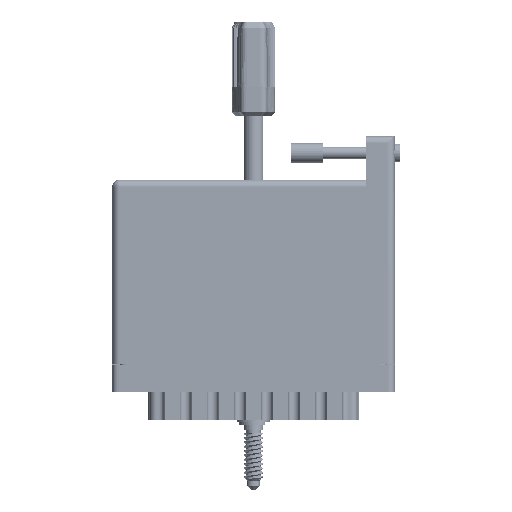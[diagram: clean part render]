
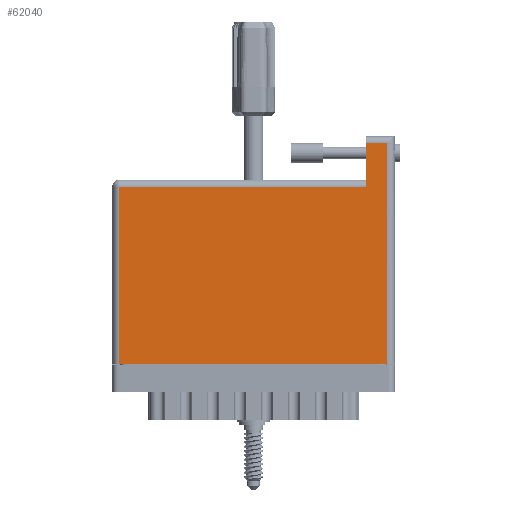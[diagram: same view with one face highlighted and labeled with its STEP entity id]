
A CAD part, front view. The second image highlights one B-rep face of the part: STEP entity #62040.
In plain terms, the highlighted face is planar.
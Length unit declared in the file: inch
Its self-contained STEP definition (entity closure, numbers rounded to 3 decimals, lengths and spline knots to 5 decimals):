
#1843 = LINE ( 'NONE', #53933, #72961 ) ;
#3958 = VERTEX_POINT ( 'NONE', #17816 ) ;
#4711 = VECTOR ( 'NONE', #77707, 39.37008 ) ;
#5452 = LINE ( 'NONE', #44135, #77604 ) ;
#7890 = CARTESIAN_POINT ( 'NONE',  ( 0., 1.775, 0. ) ) ;
#7908 = VECTOR ( 'NONE', #14143, 39.37008 ) ;
#7951 = LINE ( 'NONE', #14470, #43475 ) ;
#9631 = EDGE_CURVE ( 'NONE', #58640, #10174, #5452, .T. ) ;
#10076 = LINE ( 'NONE', #42777, #7908 ) ;
#10174 = VERTEX_POINT ( 'NONE', #40898 ) ;
#12163 = CARTESIAN_POINT ( 'NONE',  ( 2.648, 0., 0. ) ) ;
#14143 = DIRECTION ( 'NONE',  ( -1., 0., 0. ) ) ;
#14470 = CARTESIAN_POINT ( 'NONE',  ( 2.438, 2.195, 0. ) ) ;
#17816 = CARTESIAN_POINT ( 'NONE',  ( 2.438, 2.125, 0. ) ) ;
#17853 = AXIS2_PLACEMENT_3D ( 'NONE', #7890, #41314, #27472 ) ;
#20878 = LINE ( 'NONE', #71694, #4711 ) ;
#25406 = VERTEX_POINT ( 'NONE', #12163 ) ;
#27472 = DIRECTION ( 'NONE',  ( -1., 0., 0. ) ) ;
#27794 = ORIENTED_EDGE ( 'NONE', *, *, #43831, .T. ) ;
#31403 = EDGE_CURVE ( 'NONE', #37777, #58640, #10076, .T. ) ;
#35736 = CARTESIAN_POINT ( 'NONE',  ( 2.648, 2.125, 0. ) ) ;
#36382 = EDGE_CURVE ( 'NONE', #63405, #3958, #20878, .T. ) ;
#37777 = VERTEX_POINT ( 'NONE', #45306 ) ;
#40898 = CARTESIAN_POINT ( 'NONE',  ( 0.07, 0., 0. ) ) ;
#41314 = DIRECTION ( 'NONE',  ( 0., 0., -1. ) ) ;
#42777 = CARTESIAN_POINT ( 'NONE',  ( 0., 1.705, 0. ) ) ;
#43117 = FACE_OUTER_BOUND ( 'NONE', #64980, .T. ) ;
#43475 = VECTOR ( 'NONE', #55741, 39.37008 ) ;
#43831 = EDGE_CURVE ( 'NONE', #3958, #37777, #7951, .T. ) ;
#44135 = CARTESIAN_POINT ( 'NONE',  ( 0.07, 0., 0. ) ) ;
#45306 = CARTESIAN_POINT ( 'NONE',  ( 2.438, 1.705, 0. ) ) ;
#49825 = ORIENTED_EDGE ( 'NONE', *, *, #9631, .T. ) ;
#51878 = DIRECTION ( 'NONE',  ( 0., 1., 0. ) ) ;
#53933 = CARTESIAN_POINT ( 'NONE',  ( 0., 0., 0. ) ) ;
#55741 = DIRECTION ( 'NONE',  ( 0., -1., 0. ) ) ;
#57926 = DIRECTION ( 'NONE',  ( 0., -1., 0. ) ) ;
#58640 = VERTEX_POINT ( 'NONE', #62967 ) ;
#62040 = ADVANCED_FACE ( 'NONE', ( #43117 ), #69607, .F. ) ;
#62967 = CARTESIAN_POINT ( 'NONE',  ( 0.07, 1.705, 0. ) ) ;
#63405 = VERTEX_POINT ( 'NONE', #35736 ) ;
#63623 = ORIENTED_EDGE ( 'NONE', *, *, #73293, .T. ) ;
#64980 = EDGE_LOOP ( 'NONE', ( #83789, #49825, #63623, #77689, #68347, #27794 ) ) ;
#68347 = ORIENTED_EDGE ( 'NONE', *, *, #36382, .T. ) ;
#69607 = PLANE ( 'NONE',  #17853 ) ;
#71694 = CARTESIAN_POINT ( 'NONE',  ( 0., 2.125, 0. ) ) ;
#71730 = VECTOR ( 'NONE', #51878, 39.37008 ) ;
#72961 = VECTOR ( 'NONE', #81941, 39.37008 ) ;
#73293 = EDGE_CURVE ( 'NONE', #10174, #25406, #1843, .T. ) ;
#76004 = LINE ( 'NONE', #79254, #71730 ) ;
#77604 = VECTOR ( 'NONE', #57926, 39.37008 ) ;
#77689 = ORIENTED_EDGE ( 'NONE', *, *, #79903, .T. ) ;
#77707 = DIRECTION ( 'NONE',  ( -1., 0., 0. ) ) ;
#79254 = CARTESIAN_POINT ( 'NONE',  ( 2.648, 2.195, 0. ) ) ;
#79903 = EDGE_CURVE ( 'NONE', #25406, #63405, #76004, .T. ) ;
#81941 = DIRECTION ( 'NONE',  ( 1., 0., 0. ) ) ;
#83789 = ORIENTED_EDGE ( 'NONE', *, *, #31403, .T. ) ;
